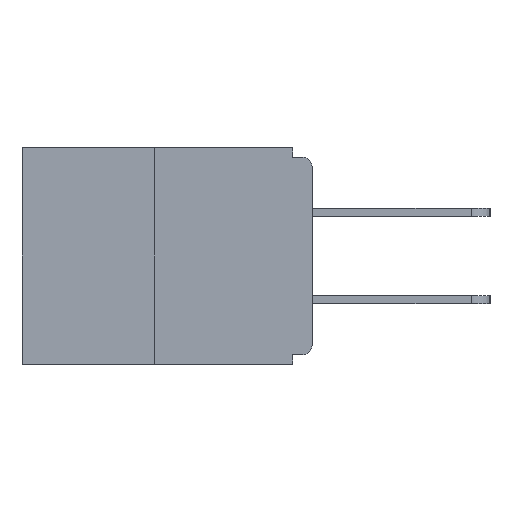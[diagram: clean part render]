
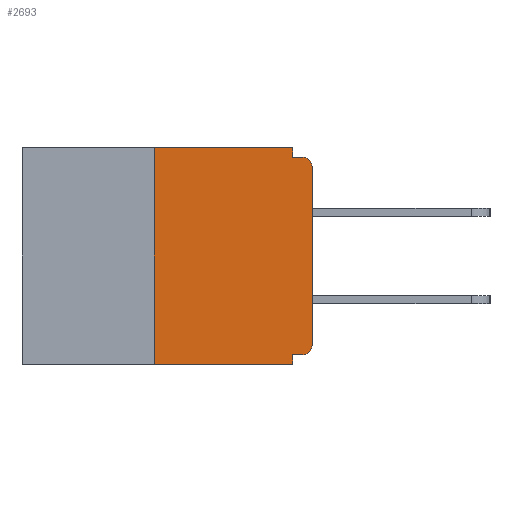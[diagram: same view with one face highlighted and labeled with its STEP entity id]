
A CAD part, left-side view. The second image highlights one B-rep face of the part: STEP entity #2693.
In plain terms, the highlighted planar face has unit normal (-1, 0, 0).
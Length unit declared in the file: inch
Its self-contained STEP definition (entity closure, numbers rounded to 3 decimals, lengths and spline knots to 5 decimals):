
#295 = DIRECTION ( 'NONE',  ( 1., 0., 0. ) ) ;
#370 = EDGE_LOOP ( 'NONE', ( #1552, #12127, #7797, #1932, #10289, #9144, #5487, #11133, #4426, #11069 ) ) ;
#387 = PLANE ( 'NONE',  #13204 ) ;
#765 = DIRECTION ( 'NONE',  ( 0., -1., 0. ) ) ;
#830 = FACE_OUTER_BOUND ( 'NONE', #370, .T. ) ;
#877 = LINE ( 'NONE', #5120, #5923 ) ;
#1273 = VECTOR ( 'NONE', #1817, 39.37008 ) ;
#1445 = EDGE_CURVE ( 'NONE', #4744, #11421, #2881, .T. ) ;
#1453 = VERTEX_POINT ( 'NONE', #7929 ) ;
#1479 = CARTESIAN_POINT ( 'NONE',  ( 0., 0.031, 0. ) ) ;
#1491 = LINE ( 'NONE', #8035, #6894 ) ;
#1552 = ORIENTED_EDGE ( 'NONE', *, *, #6266, .F. ) ;
#1573 = LINE ( 'NONE', #3219, #13264 ) ;
#1813 = CARTESIAN_POINT ( 'NONE',  ( 0., 0., -0.313 ) ) ;
#1817 = DIRECTION ( 'NONE',  ( 0., 0., -1. ) ) ;
#1836 = CARTESIAN_POINT ( 'NONE',  ( 0., 0.015, -0.328 ) ) ;
#1932 = ORIENTED_EDGE ( 'NONE', *, *, #6336, .F. ) ;
#1938 = LINE ( 'NONE', #12550, #1273 ) ;
#2388 = CARTESIAN_POINT ( 'NONE',  ( 0., 0.015, -0.313 ) ) ;
#2470 = CARTESIAN_POINT ( 'NONE',  ( 0., 0., -0.328 ) ) ;
#2588 = DIRECTION ( 'NONE',  ( 0., 0., -1. ) ) ;
#2677 = CARTESIAN_POINT ( 'NONE',  ( 0., 0.031, -0.328 ) ) ;
#2693 = ADVANCED_FACE ( 'NONE', ( #830 ), #387, .F. ) ;
#2707 = VECTOR ( 'NONE', #6908, 39.37008 ) ;
#2858 = DIRECTION ( 'NONE',  ( 0., 0., 1. ) ) ;
#2881 = LINE ( 'NONE', #2470, #2707 ) ;
#3097 = EDGE_CURVE ( 'NONE', #4464, #12388, #1491, .T. ) ;
#3219 = CARTESIAN_POINT ( 'NONE',  ( 0., 0.031, -0.343 ) ) ;
#3336 = CARTESIAN_POINT ( 'NONE',  ( 0., 0.25, -0.343 ) ) ;
#3700 = DIRECTION ( 'NONE',  ( 0., -1., 0. ) ) ;
#3971 = CIRCLE ( 'NONE', #13930, 0.015 ) ;
#4153 = EDGE_CURVE ( 'NONE', #13802, #5483, #10418, .T. ) ;
#4426 = ORIENTED_EDGE ( 'NONE', *, *, #12976, .F. ) ;
#4464 = VERTEX_POINT ( 'NONE', #3336 ) ;
#4744 = VERTEX_POINT ( 'NONE', #1836 ) ;
#4942 = VECTOR ( 'NONE', #765, 39.37008 ) ;
#5120 = CARTESIAN_POINT ( 'NONE',  ( 0., 0.25, 0. ) ) ;
#5342 = AXIS2_PLACEMENT_3D ( 'NONE', #10149, #10103, #2588 ) ;
#5419 = CARTESIAN_POINT ( 'NONE',  ( 0., 0., 0. ) ) ;
#5450 = LINE ( 'NONE', #11617, #4942 ) ;
#5483 = VERTEX_POINT ( 'NONE', #13126 ) ;
#5487 = ORIENTED_EDGE ( 'NONE', *, *, #4153, .T. ) ;
#5923 = VECTOR ( 'NONE', #2858, 39.37008 ) ;
#5944 = CARTESIAN_POINT ( 'NONE',  ( 0., 0.031, -0.343 ) ) ;
#5958 = CARTESIAN_POINT ( 'NONE',  ( 0., 0.25, 0. ) ) ;
#6067 = VERTEX_POINT ( 'NONE', #1479 ) ;
#6266 = EDGE_CURVE ( 'NONE', #10975, #6067, #5450, .T. ) ;
#6336 = EDGE_CURVE ( 'NONE', #11421, #12388, #1573, .T. ) ;
#6413 = DIRECTION ( 'NONE',  ( 0., 0., -1. ) ) ;
#6443 = CARTESIAN_POINT ( 'NONE',  ( 0., 0.015, -0.015 ) ) ;
#6810 = EDGE_CURVE ( 'NONE', #5483, #10927, #9364, .T. ) ;
#6894 = VECTOR ( 'NONE', #3700, 39.37008 ) ;
#6908 = DIRECTION ( 'NONE',  ( 0., 1., 0. ) ) ;
#7717 = DIRECTION ( 'NONE',  ( 0., 0., -1. ) ) ;
#7797 = ORIENTED_EDGE ( 'NONE', *, *, #3097, .T. ) ;
#7929 = CARTESIAN_POINT ( 'NONE',  ( 0., 0.031, -0.015 ) ) ;
#8035 = CARTESIAN_POINT ( 'NONE',  ( 0., 0.46, -0.343 ) ) ;
#8873 = CARTESIAN_POINT ( 'NONE',  ( 0., 0.46, 0. ) ) ;
#9045 = EDGE_CURVE ( 'NONE', #4744, #13802, #3971, .T. ) ;
#9144 = ORIENTED_EDGE ( 'NONE', *, *, #9045, .T. ) ;
#9315 = EDGE_CURVE ( 'NONE', #6067, #1453, #1938, .T. ) ;
#9364 = CIRCLE ( 'NONE', #5342, 0.015 ) ;
#9957 = LINE ( 'NONE', #10257, #11820 ) ;
#9966 = DIRECTION ( 'NONE',  ( 0., 0., -1. ) ) ;
#10103 = DIRECTION ( 'NONE',  ( -1., 0., 0. ) ) ;
#10149 = CARTESIAN_POINT ( 'NONE',  ( 0., 0.015, -0.03 ) ) ;
#10257 = CARTESIAN_POINT ( 'NONE',  ( 0., 0., -0.015 ) ) ;
#10289 = ORIENTED_EDGE ( 'NONE', *, *, #1445, .F. ) ;
#10418 = LINE ( 'NONE', #5419, #12449 ) ;
#10845 = EDGE_CURVE ( 'NONE', #4464, #10975, #877, .T. ) ;
#10927 = VERTEX_POINT ( 'NONE', #6443 ) ;
#10975 = VERTEX_POINT ( 'NONE', #5958 ) ;
#11069 = ORIENTED_EDGE ( 'NONE', *, *, #9315, .F. ) ;
#11133 = ORIENTED_EDGE ( 'NONE', *, *, #6810, .T. ) ;
#11420 = DIRECTION ( 'NONE',  ( 0., -1., 0. ) ) ;
#11421 = VERTEX_POINT ( 'NONE', #2677 ) ;
#11617 = CARTESIAN_POINT ( 'NONE',  ( 0., 0.46, 0. ) ) ;
#11820 = VECTOR ( 'NONE', #11420, 39.37008 ) ;
#12126 = DIRECTION ( 'NONE',  ( -1., 0., 0. ) ) ;
#12127 = ORIENTED_EDGE ( 'NONE', *, *, #10845, .F. ) ;
#12388 = VERTEX_POINT ( 'NONE', #5944 ) ;
#12449 = VECTOR ( 'NONE', #13016, 39.37008 ) ;
#12550 = CARTESIAN_POINT ( 'NONE',  ( 0., 0.031, 0. ) ) ;
#12976 = EDGE_CURVE ( 'NONE', #1453, #10927, #9957, .T. ) ;
#13016 = DIRECTION ( 'NONE',  ( 0., 0., 1. ) ) ;
#13126 = CARTESIAN_POINT ( 'NONE',  ( 0., 0., -0.03 ) ) ;
#13204 = AXIS2_PLACEMENT_3D ( 'NONE', #8873, #295, #9966 ) ;
#13264 = VECTOR ( 'NONE', #6413, 39.37008 ) ;
#13802 = VERTEX_POINT ( 'NONE', #1813 ) ;
#13930 = AXIS2_PLACEMENT_3D ( 'NONE', #2388, #12126, #7717 ) ;
